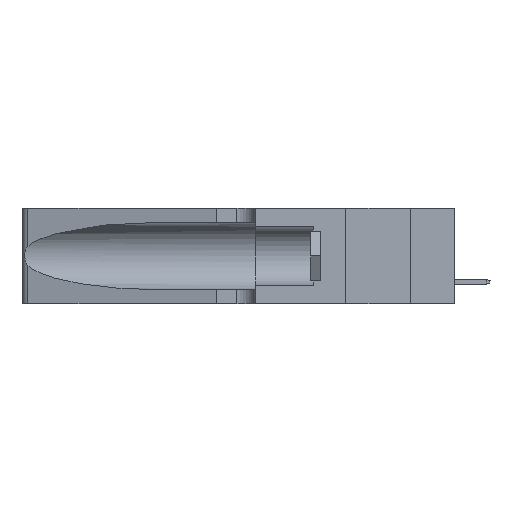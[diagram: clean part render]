
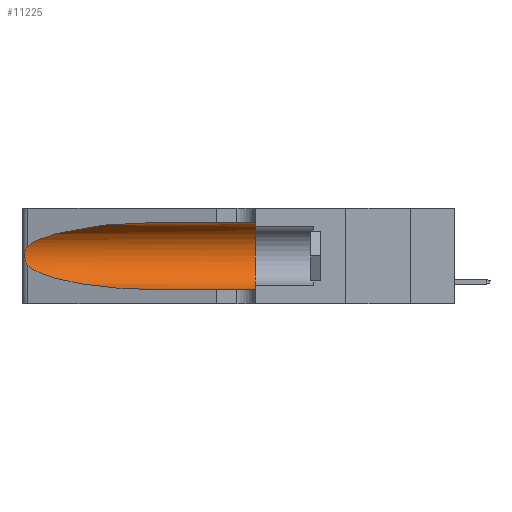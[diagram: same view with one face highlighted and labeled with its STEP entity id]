
A CAD part, left-side view. The second image highlights one B-rep face of the part: STEP entity #11225.
In plain terms, the highlighted cylindrical face has radius 3.308 mm (diameter 6.617 mm), a partial arc.
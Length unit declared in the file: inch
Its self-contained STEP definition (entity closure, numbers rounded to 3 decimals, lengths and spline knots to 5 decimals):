
#888 = CARTESIAN_POINT ( 'NONE',  ( 0.25487, 1.22718, 0.14631 ) ) ;
#1395 = ORIENTED_EDGE ( 'NONE', *, *, #14820, .T. ) ;
#2685 = EDGE_CURVE ( 'NONE', #34747, #21567, #19404, .T. ) ;
#4397 = VERTEX_POINT ( 'NONE', #28182 ) ;
#5163 = DIRECTION ( 'NONE',  ( 0., -1., 0. ) ) ;
#5464 = VERTEX_POINT ( 'NONE', #20735 ) ;
#5640 = ORIENTED_EDGE ( 'NONE', *, *, #35214, .T. ) ;
#6224 = ORIENTED_EDGE ( 'NONE', *, *, #11955, .T. ) ;
#6788 = CARTESIAN_POINT ( 'NONE',  ( 0.25854, 1.2359, 0.20912 ) ) ;
#6851 = CARTESIAN_POINT ( 'NONE',  ( 0.25487, 1.22718, 0.22369 ) ) ;
#7027 = DIRECTION ( 'NONE',  ( 0., 0., 1. ) ) ;
#7061 = B_SPLINE_CURVE_WITH_KNOTS ( 'NONE', 3,
 ( #24031, #7152, #18415, #12984, #6788, #12792, #9968, #18767, #21393, #30398, #13346, #35485, #9786, #24208 ),
 .UNSPECIFIED., .F., .F.,
 ( 4, 2, 2, 2, 2, 2, 4 ),
 ( 0., 0.00027, 0.00053, 0.00107, 0.0016, 0.00187, 0.00214 ),
 .UNSPECIFIED. ) ;
#7152 = CARTESIAN_POINT ( 'NONE',  ( 0.25555, 1.22994, 0.2215 ) ) ;
#7930 = CARTESIAN_POINT ( 'NONE',  ( 0.1305, 0.72297, 0.05475 ) ) ;
#9361 = AXIS2_PLACEMENT_3D ( 'NONE', #11599, #20578, #32413 ) ;
#9681 = EDGE_LOOP ( 'NONE', ( #5640, #1395, #24196, #6224, #11433, #29660 ) ) ;
#9786 = CARTESIAN_POINT ( 'NONE',  ( 0.25555, 1.22993, 0.14849 ) ) ;
#9968 = CARTESIAN_POINT ( 'NONE',  ( 0.26075, 1.23896, 0.19203 ) ) ;
#11225 = ADVANCED_FACE ( 'NONE', ( #20962 ), #28846, .F. ) ;
#11433 = ORIENTED_EDGE ( 'NONE', *, *, #11769, .F. ) ;
#11507 = CARTESIAN_POINT ( 'NONE',  ( 0.1305, 1.61858, 0.05475 ) ) ;
#11599 = CARTESIAN_POINT ( 'NONE',  ( 0.1305, 1.61858, 0.185 ) ) ;
#11769 = EDGE_CURVE ( 'NONE', #21567, #5464, #22584, .T. ) ;
#11955 = EDGE_CURVE ( 'NONE', #16327, #5464, #32135, .T. ) ;
#12792 = CARTESIAN_POINT ( 'NONE',  ( 0.26018, 1.23835, 0.19895 ) ) ;
#12984 = CARTESIAN_POINT ( 'NONE',  ( 0.25787, 1.23484, 0.2124 ) ) ;
#13346 = CARTESIAN_POINT ( 'NONE',  ( 0.25789, 1.23486, 0.15765 ) ) ;
#14294 = VECTOR ( 'NONE', #5163, 39.37008 ) ;
#14820 = EDGE_CURVE ( 'NONE', #24620, #4397, #7061, .T. ) ;
#15343 = CARTESIAN_POINT ( 'NONE',  ( 0.18966, 0.96281, 0.05475 ) ) ;
#15502 = CARTESIAN_POINT ( 'NONE',  ( 0.1305, 0.35, 0.185 ) ) ;
#16327 = VERTEX_POINT ( 'NONE', #7930 ) ;
#16698 = CARTESIAN_POINT ( 'NONE',  ( 0.2373, 1.15595, 0.28018 ) ) ;
#16700 = CARTESIAN_POINT ( 'NONE',  ( 0.1305, 0.35, 0.31525 ) ) ;
#18415 = CARTESIAN_POINT ( 'NONE',  ( 0.25639, 1.23184, 0.21858 ) ) ;
#18767 = CARTESIAN_POINT ( 'NONE',  ( 0.26075, 1.23896, 0.178 ) ) ;
#19295 =( BOUNDED_CURVE ( )  B_SPLINE_CURVE ( 3, ( #888, #20756, #15343, #27116 ),
 .UNSPECIFIED., .F., .F. ) 
 B_SPLINE_CURVE_WITH_KNOTS ( ( 4, 4 ),
 ( 3.44316, 4.71239 ),
 .UNSPECIFIED. ) 
 CURVE ( )  GEOMETRIC_REPRESENTATION_ITEM ( )  RATIONAL_B_SPLINE_CURVE ( ( 1., 0.87, 0.87, 1. ) ) 
 REPRESENTATION_ITEM ( '' )  );
#19404 = LINE ( 'NONE', #30848, #14294 ) ;
#19863 = CARTESIAN_POINT ( 'NONE',  ( 0.1305, 0.72297, 0.31525 ) ) ;
#20578 = DIRECTION ( 'NONE',  ( 0., -1., 0. ) ) ;
#20735 = CARTESIAN_POINT ( 'NONE',  ( 0.1305, 0.35, 0.05475 ) ) ;
#20756 = CARTESIAN_POINT ( 'NONE',  ( 0.2373, 1.15595, 0.08982 ) ) ;
#20962 = FACE_OUTER_BOUND ( 'NONE', #9681, .T. ) ;
#21393 = CARTESIAN_POINT ( 'NONE',  ( 0.26017, 1.23833, 0.17102 ) ) ;
#21567 = VERTEX_POINT ( 'NONE', #16700 ) ;
#22117 = CARTESIAN_POINT ( 'NONE',  ( 0.25487, 1.22718, 0.22369 ) ) ;
#22584 = CIRCLE ( 'NONE', #29757, 0.13025 ) ;
#24031 = CARTESIAN_POINT ( 'NONE',  ( 0.25487, 1.22718, 0.22369 ) ) ;
#24105 =( BOUNDED_CURVE ( )  B_SPLINE_CURVE ( 3, ( #19863, #33762, #16698, #22117 ),
 .UNSPECIFIED., .F., .F. ) 
 B_SPLINE_CURVE_WITH_KNOTS ( ( 4, 4 ),
 ( 1.5708, 2.84003 ),
 .UNSPECIFIED. ) 
 CURVE ( )  GEOMETRIC_REPRESENTATION_ITEM ( )  RATIONAL_B_SPLINE_CURVE ( ( 1., 0.87, 0.87, 1. ) ) 
 REPRESENTATION_ITEM ( '' )  );
#24196 = ORIENTED_EDGE ( 'NONE', *, *, #30599, .T. ) ;
#24208 = CARTESIAN_POINT ( 'NONE',  ( 0.25487, 1.22718, 0.14631 ) ) ;
#24272 = DIRECTION ( 'NONE',  ( 0., 1., 0. ) ) ;
#24620 = VERTEX_POINT ( 'NONE', #6851 ) ;
#27116 = CARTESIAN_POINT ( 'NONE',  ( 0.1305, 0.72297, 0.05475 ) ) ;
#28182 = CARTESIAN_POINT ( 'NONE',  ( 0.25487, 1.22718, 0.14631 ) ) ;
#28846 = CYLINDRICAL_SURFACE ( 'NONE', #9361, 0.13025 ) ;
#29660 = ORIENTED_EDGE ( 'NONE', *, *, #2685, .F. ) ;
#29757 = AXIS2_PLACEMENT_3D ( 'NONE', #15502, #24272, #7027 ) ;
#30398 = CARTESIAN_POINT ( 'NONE',  ( 0.25856, 1.23593, 0.16098 ) ) ;
#30599 = EDGE_CURVE ( 'NONE', #4397, #16327, #19295, .T. ) ;
#30848 = CARTESIAN_POINT ( 'NONE',  ( 0.1305, 1.61858, 0.31525 ) ) ;
#32135 = LINE ( 'NONE', #11507, #35761 ) ;
#32413 = DIRECTION ( 'NONE',  ( 0., 0., -1. ) ) ;
#33619 = CARTESIAN_POINT ( 'NONE',  ( 0.1305, 0.72297, 0.31525 ) ) ;
#33762 = CARTESIAN_POINT ( 'NONE',  ( 0.18966, 0.96281, 0.31525 ) ) ;
#34747 = VERTEX_POINT ( 'NONE', #33619 ) ;
#35214 = EDGE_CURVE ( 'NONE', #34747, #24620, #24105, .T. ) ;
#35485 = CARTESIAN_POINT ( 'NONE',  ( 0.25639, 1.23186, 0.15144 ) ) ;
#35761 = VECTOR ( 'NONE', #37038, 39.37008 ) ;
#37038 = DIRECTION ( 'NONE',  ( 0., -1., 0. ) ) ;
